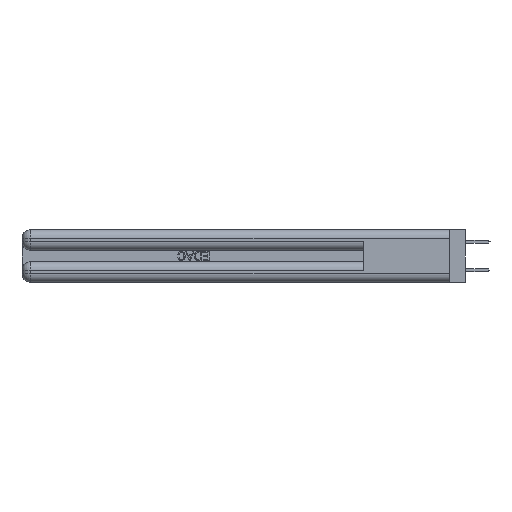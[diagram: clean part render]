
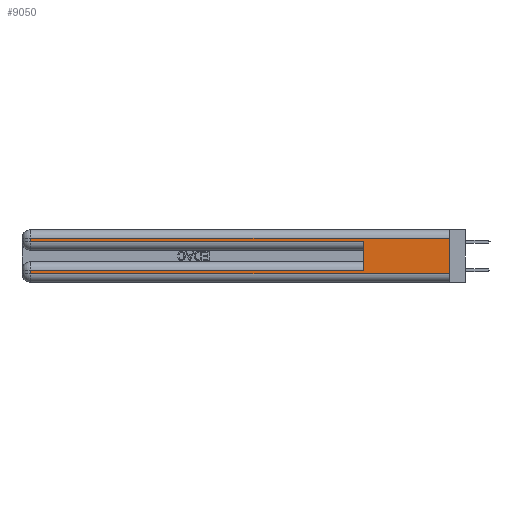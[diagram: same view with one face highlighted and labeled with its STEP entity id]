
A CAD part, left-side view. The second image highlights one B-rep face of the part: STEP entity #9050.
In plain terms, the highlighted planar face has unit normal (-1, 0, 0).
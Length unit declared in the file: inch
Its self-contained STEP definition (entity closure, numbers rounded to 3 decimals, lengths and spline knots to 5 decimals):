
#242 = VECTOR ( 'NONE', #12468, 39.37008 ) ;
#715 = CARTESIAN_POINT ( 'NONE',  ( 0., 0., 0.37 ) ) ;
#1127 = CARTESIAN_POINT ( 'NONE',  ( 0., 2.94, 0.06 ) ) ;
#1210 = VECTOR ( 'NONE', #23760, 39.37008 ) ;
#1381 = PLANE ( 'NONE',  #12064 ) ;
#2285 = VERTEX_POINT ( 'NONE', #16167 ) ;
#2634 = CARTESIAN_POINT ( 'NONE',  ( 0., 0., 0.06 ) ) ;
#2839 = CARTESIAN_POINT ( 'NONE',  ( 0., 0.6, 0.285 ) ) ;
#3359 = VERTEX_POINT ( 'NONE', #27821 ) ;
#3525 = VECTOR ( 'NONE', #24703, 39.37008 ) ;
#3777 = DIRECTION ( 'NONE',  ( 1., 0., 0. ) ) ;
#3876 = VECTOR ( 'NONE', #39942, 39.37008 ) ;
#3904 = EDGE_CURVE ( 'NONE', #2285, #35444, #19814, .T. ) ;
#4230 = LINE ( 'NONE', #39824, #40061 ) ;
#5247 = EDGE_CURVE ( 'NONE', #17908, #24339, #13149, .T. ) ;
#5385 = LINE ( 'NONE', #6613, #32876 ) ;
#5510 = ORIENTED_EDGE ( 'NONE', *, *, #22995, .F. ) ;
#6613 = CARTESIAN_POINT ( 'NONE',  ( 0., 0.6, 0.145 ) ) ;
#6759 = DIRECTION ( 'NONE',  ( 0., 0., 1. ) ) ;
#9050 = ADVANCED_FACE ( 'NONE', ( #14820 ), #1381, .F. ) ;
#9245 = LINE ( 'NONE', #23351, #9762 ) ;
#9731 = VERTEX_POINT ( 'NONE', #43310 ) ;
#9762 = VECTOR ( 'NONE', #40365, 39.37008 ) ;
#10767 = EDGE_CURVE ( 'NONE', #2285, #3359, #9245, .T. ) ;
#11814 = VECTOR ( 'NONE', #26060, 39.37008 ) ;
#12064 = AXIS2_PLACEMENT_3D ( 'NONE', #715, #3777, #21230 ) ;
#12127 = EDGE_CURVE ( 'NONE', #35109, #35444, #40568, .T. ) ;
#12468 = DIRECTION ( 'NONE',  ( 0., 0., -1. ) ) ;
#12629 = CARTESIAN_POINT ( 'NONE',  ( 0., 2.94, 0.285 ) ) ;
#13149 = LINE ( 'NONE', #44556, #1210 ) ;
#14820 = FACE_OUTER_BOUND ( 'NONE', #39199, .T. ) ;
#15809 = CARTESIAN_POINT ( 'NONE',  ( 0., 2.94, 0.37 ) ) ;
#16167 = CARTESIAN_POINT ( 'NONE',  ( 0., 0., 0.31 ) ) ;
#16772 = CARTESIAN_POINT ( 'NONE',  ( 0., 0.6, 0.085 ) ) ;
#17908 = VERTEX_POINT ( 'NONE', #12629 ) ;
#19814 = LINE ( 'NONE', #38538, #3525 ) ;
#20168 = ORIENTED_EDGE ( 'NONE', *, *, #32101, .T. ) ;
#20905 = LINE ( 'NONE', #15809, #242 ) ;
#21230 = DIRECTION ( 'NONE',  ( 0., 0., -1. ) ) ;
#21899 = ORIENTED_EDGE ( 'NONE', *, *, #10767, .T. ) ;
#21901 = ORIENTED_EDGE ( 'NONE', *, *, #5247, .T. ) ;
#22995 = EDGE_CURVE ( 'NONE', #24924, #24339, #5385, .T. ) ;
#23282 = ORIENTED_EDGE ( 'NONE', *, *, #25838, .T. ) ;
#23351 = CARTESIAN_POINT ( 'NONE',  ( 0., 0., 0.31 ) ) ;
#23760 = DIRECTION ( 'NONE',  ( 0., -1., 0. ) ) ;
#24339 = VERTEX_POINT ( 'NONE', #2839 ) ;
#24703 = DIRECTION ( 'NONE',  ( 0., 0., -1. ) ) ;
#24924 = VERTEX_POINT ( 'NONE', #16772 ) ;
#25838 = EDGE_CURVE ( 'NONE', #3359, #17908, #20905, .T. ) ;
#26060 = DIRECTION ( 'NONE',  ( 0., -1., 0. ) ) ;
#27767 = ORIENTED_EDGE ( 'NONE', *, *, #12127, .T. ) ;
#27821 = CARTESIAN_POINT ( 'NONE',  ( 0., 2.94, 0.31 ) ) ;
#29829 = ORIENTED_EDGE ( 'NONE', *, *, #3904, .F. ) ;
#30230 = CARTESIAN_POINT ( 'NONE',  ( 0., 0., 0.085 ) ) ;
#31008 = ORIENTED_EDGE ( 'NONE', *, *, #43418, .T. ) ;
#32101 = EDGE_CURVE ( 'NONE', #9731, #35109, #4230, .T. ) ;
#32876 = VECTOR ( 'NONE', #6759, 39.37008 ) ;
#35109 = VERTEX_POINT ( 'NONE', #1127 ) ;
#35444 = VERTEX_POINT ( 'NONE', #2634 ) ;
#38538 = CARTESIAN_POINT ( 'NONE',  ( 0., 0., 0.37 ) ) ;
#39199 = EDGE_LOOP ( 'NONE', ( #29829, #21899, #23282, #21901, #5510, #31008, #20168, #27767 ) ) ;
#39824 = CARTESIAN_POINT ( 'NONE',  ( 0., 2.94, 0.37 ) ) ;
#39942 = DIRECTION ( 'NONE',  ( 0., 1., 0. ) ) ;
#40061 = VECTOR ( 'NONE', #40138, 39.37008 ) ;
#40138 = DIRECTION ( 'NONE',  ( 0., 0., -1. ) ) ;
#40365 = DIRECTION ( 'NONE',  ( 0., 1., 0. ) ) ;
#40568 = LINE ( 'NONE', #42247, #11814 ) ;
#41313 = LINE ( 'NONE', #30230, #3876 ) ;
#42247 = CARTESIAN_POINT ( 'NONE',  ( 0., 0., 0.06 ) ) ;
#43310 = CARTESIAN_POINT ( 'NONE',  ( 0., 2.94, 0.085 ) ) ;
#43418 = EDGE_CURVE ( 'NONE', #24924, #9731, #41313, .T. ) ;
#44556 = CARTESIAN_POINT ( 'NONE',  ( 0., 0., 0.285 ) ) ;
